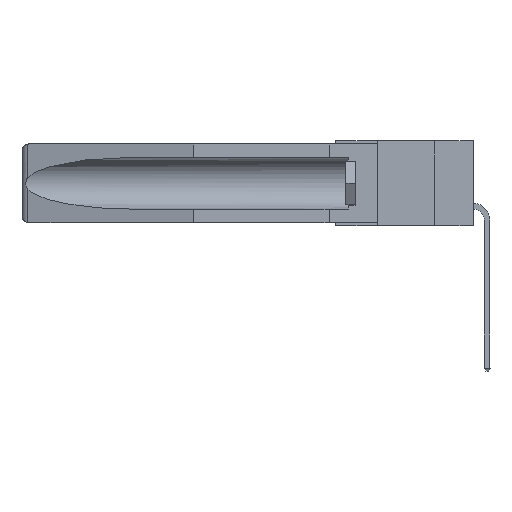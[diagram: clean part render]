
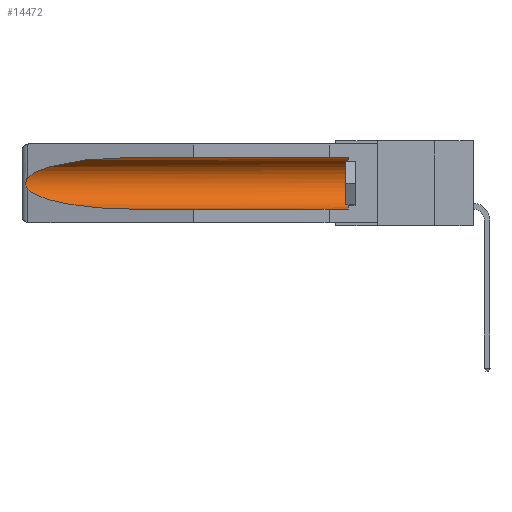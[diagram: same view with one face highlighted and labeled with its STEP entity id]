
A CAD part, left-side view. The second image highlights one B-rep face of the part: STEP entity #14472.
In plain terms, the highlighted cylindrical face has radius 2.857 mm (diameter 5.715 mm), a partial arc.
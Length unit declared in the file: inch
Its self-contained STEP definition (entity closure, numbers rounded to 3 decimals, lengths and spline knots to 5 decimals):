
#494 = VECTOR ( 'NONE', #6477, 39.37008 ) ;
#1177 = EDGE_CURVE ( 'NONE', #5364, #15643, #15458, .T. ) ;
#1241 = ORIENTED_EDGE ( 'NONE', *, *, #11830, .T. ) ;
#1623 = CARTESIAN_POINT ( 'NONE',  ( 0.155, 1.07973, -0.284 ) ) ;
#1885 = B_SPLINE_CURVE_WITH_KNOTS ( 'NONE', 3,
 ( #2342, #3880, #16506, #2576, #14145, #10135, #3819, #15447, #12817, #10188 ),
 .UNSPECIFIED., .F., .F.,
 ( 4, 2, 2, 2, 4 ),
 ( 0., 0.00029, 0.00058, 0.00087, 0.00117 ),
 .UNSPECIFIED. ) ;
#2342 = CARTESIAN_POINT ( 'NONE',  ( 0.26537, 1.52718, -0.14972 ) ) ;
#2413 = VERTEX_POINT ( 'NONE', #13423 ) ;
#2576 = CARTESIAN_POINT ( 'NONE',  ( 0.2673, 1.5327, -0.16383 ) ) ;
#2668 = VERTEX_POINT ( 'NONE', #11210 ) ;
#2872 = CARTESIAN_POINT ( 'NONE',  ( 0.26537, 1.52718, -0.14972 ) ) ;
#2888 = CARTESIAN_POINT ( 'NONE',  ( 0.26537, 1.52718, -0.19328 ) ) ;
#3050 = CARTESIAN_POINT ( 'NONE',  ( 0.21114, 1.30732, -0.284 ) ) ;
#3819 = CARTESIAN_POINT ( 'NONE',  ( 0.2673, 1.53269, -0.17917 ) ) ;
#3880 = CARTESIAN_POINT ( 'NONE',  ( 0.26597, 1.52961, -0.15275 ) ) ;
#4773 = CARTESIAN_POINT ( 'NONE',  ( 0.155, 1.07973, -0.284 ) ) ;
#4907 = FACE_OUTER_BOUND ( 'NONE', #13417, .T. ) ;
#4985 = CARTESIAN_POINT ( 'NONE',  ( 0.155, 0.126, -0.1715 ) ) ;
#5275 = CARTESIAN_POINT ( 'NONE',  ( 0.155, -0.30754, -0.1715 ) ) ;
#5364 = VERTEX_POINT ( 'NONE', #11781 ) ;
#5970 = ORIENTED_EDGE ( 'NONE', *, *, #1177, .T. ) ;
#6037 = EDGE_CURVE ( 'NONE', #2668, #12676, #7609, .T. ) ;
#6226 = ORIENTED_EDGE ( 'NONE', *, *, #11878, .T. ) ;
#6477 = DIRECTION ( 'NONE',  ( 0., 1., 0. ) ) ;
#6961 = ORIENTED_EDGE ( 'NONE', *, *, #15415, .T. ) ;
#7078 = VECTOR ( 'NONE', #16347, 39.37008 ) ;
#7579 = DIRECTION ( 'NONE',  ( 0., 0., 1. ) ) ;
#7609 =( BOUNDED_CURVE ( )  B_SPLINE_CURVE ( 3, ( #2888, #10770, #3050, #1623 ),
 .UNSPECIFIED., .F., .F. ) 
 B_SPLINE_CURVE_WITH_KNOTS ( ( 4, 4 ),
 ( 0.1948, 1.5708 ),
 .UNSPECIFIED. ) 
 CURVE ( )  GEOMETRIC_REPRESENTATION_ITEM ( )  RATIONAL_B_SPLINE_CURVE ( ( 1., 0.848, 0.848, 1. ) ) 
 REPRESENTATION_ITEM ( '' )  );
#7684 = ORIENTED_EDGE ( 'NONE', *, *, #15044, .F. ) ;
#7895 = CARTESIAN_POINT ( 'NONE',  ( 0.25451, 1.48313, -0.09465 ) ) ;
#8127 = ORIENTED_EDGE ( 'NONE', *, *, #6037, .T. ) ;
#9157 = VERTEX_POINT ( 'NONE', #9927 ) ;
#9719 = AXIS2_PLACEMENT_3D ( 'NONE', #5275, #11690, #12900 ) ;
#9927 = CARTESIAN_POINT ( 'NONE',  ( 0.26537, 1.52718, -0.14972 ) ) ;
#10062 = CARTESIAN_POINT ( 'NONE',  ( 0.155, 0.126, -0.059 ) ) ;
#10135 = CARTESIAN_POINT ( 'NONE',  ( 0.2675, 1.53308, -0.17534 ) ) ;
#10188 = CARTESIAN_POINT ( 'NONE',  ( 0.26537, 1.52718, -0.19328 ) ) ;
#10770 = CARTESIAN_POINT ( 'NONE',  ( 0.25451, 1.48313, -0.24835 ) ) ;
#11210 = CARTESIAN_POINT ( 'NONE',  ( 0.26537, 1.52718, -0.19328 ) ) ;
#11690 = DIRECTION ( 'NONE',  ( 0., 1., 0. ) ) ;
#11781 = CARTESIAN_POINT ( 'NONE',  ( 0.155, 0.126, -0.284 ) ) ;
#11830 = EDGE_CURVE ( 'NONE', #15643, #2413, #15874, .T. ) ;
#11878 = EDGE_CURVE ( 'NONE', #9157, #2668, #1885, .T. ) ;
#12676 = VERTEX_POINT ( 'NONE', #4773 ) ;
#12817 = CARTESIAN_POINT ( 'NONE',  ( 0.26597, 1.5296, -0.19026 ) ) ;
#12900 = DIRECTION ( 'NONE',  ( 0., 0., 1. ) ) ;
#13303 = CYLINDRICAL_SURFACE ( 'NONE', #9719, 0.1125 ) ;
#13417 = EDGE_LOOP ( 'NONE', ( #6961, #6226, #8127, #7684, #5970, #1241 ) ) ;
#13423 = CARTESIAN_POINT ( 'NONE',  ( 0.155, 1.07973, -0.059 ) ) ;
#13873 = CARTESIAN_POINT ( 'NONE',  ( 0.155, 1.07973, -0.059 ) ) ;
#14145 = CARTESIAN_POINT ( 'NONE',  ( 0.2675, 1.53308, -0.16763 ) ) ;
#14472 = ADVANCED_FACE ( 'NONE', ( #4907 ), #13303, .F. ) ;
#14491 = LINE ( 'NONE', #15404, #7078 ) ;
#14558 =( BOUNDED_CURVE ( )  B_SPLINE_CURVE ( 3, ( #13873, #16352, #7895, #2872 ),
 .UNSPECIFIED., .F., .F. ) 
 B_SPLINE_CURVE_WITH_KNOTS ( ( 4, 4 ),
 ( 4.71239, 6.08839 ),
 .UNSPECIFIED. ) 
 CURVE ( )  GEOMETRIC_REPRESENTATION_ITEM ( )  RATIONAL_B_SPLINE_CURVE ( ( 1., 0.848, 0.848, 1. ) ) 
 REPRESENTATION_ITEM ( '' )  );
#15044 = EDGE_CURVE ( 'NONE', #5364, #12676, #14491, .T. ) ;
#15247 = DIRECTION ( 'NONE',  ( 0., -1., 0. ) ) ;
#15404 = CARTESIAN_POINT ( 'NONE',  ( 0.155, -0.30754, -0.284 ) ) ;
#15415 = EDGE_CURVE ( 'NONE', #2413, #9157, #14558, .T. ) ;
#15447 = CARTESIAN_POINT ( 'NONE',  ( 0.26655, 1.53094, -0.18657 ) ) ;
#15458 = CIRCLE ( 'NONE', #16340, 0.1125 ) ;
#15643 = VERTEX_POINT ( 'NONE', #10062 ) ;
#15874 = LINE ( 'NONE', #16276, #494 ) ;
#16276 = CARTESIAN_POINT ( 'NONE',  ( 0.155, -0.30754, -0.059 ) ) ;
#16340 = AXIS2_PLACEMENT_3D ( 'NONE', #4985, #15247, #7579 ) ;
#16347 = DIRECTION ( 'NONE',  ( 0., 1., 0. ) ) ;
#16352 = CARTESIAN_POINT ( 'NONE',  ( 0.21114, 1.30732, -0.059 ) ) ;
#16506 = CARTESIAN_POINT ( 'NONE',  ( 0.26654, 1.53092, -0.15636 ) ) ;
